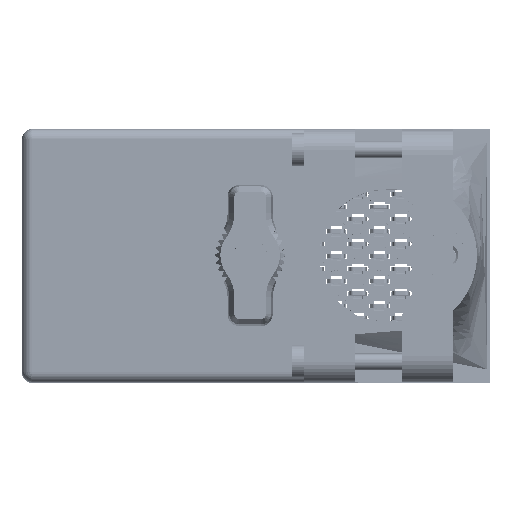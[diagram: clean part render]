
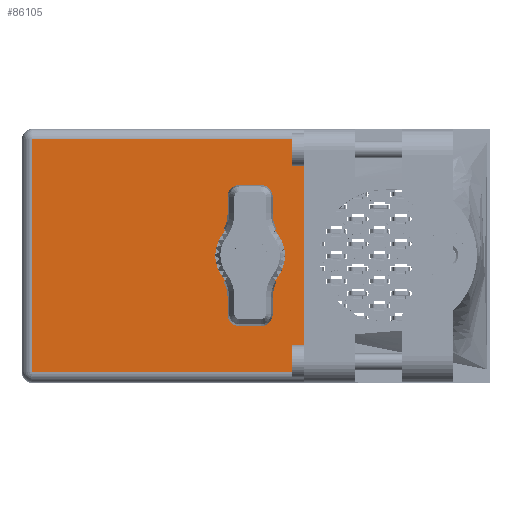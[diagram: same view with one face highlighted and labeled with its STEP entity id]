
A CAD part, top view. The second image highlights one B-rep face of the part: STEP entity #86105.
In plain terms, the highlighted face is planar.
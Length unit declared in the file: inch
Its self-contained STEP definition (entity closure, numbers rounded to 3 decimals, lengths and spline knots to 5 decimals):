
#729 = DIRECTION ( 'NONE',  ( -1., 0., 0. ) ) ;
#3442 = EDGE_CURVE ( 'NONE', #18432, #113699, #70289, .T. ) ;
#4552 = AXIS2_PLACEMENT_3D ( 'NONE', #9886, #89117, #91411 ) ;
#6389 = CIRCLE ( 'NONE', #4552, 0.17 ) ;
#8356 = EDGE_LOOP ( 'NONE', ( #48744, #97580 ) ) ;
#9886 = CARTESIAN_POINT ( 'NONE',  ( 0., 1.93, 0. ) ) ;
#10807 = CARTESIAN_POINT ( 'NONE',  ( 0., 1.93, 0.17 ) ) ;
#12747 = EDGE_CURVE ( 'NONE', #40811, #113699, #49212, .T. ) ;
#14676 = VECTOR ( 'NONE', #64042, 39.37008 ) ;
#18432 = VERTEX_POINT ( 'NONE', #103805 ) ;
#19051 = EDGE_CURVE ( 'NONE', #43180, #21117, #98199, .T. ) ;
#19442 = AXIS2_PLACEMENT_3D ( 'NONE', #82333, #20128, #91129 ) ;
#19872 = EDGE_CURVE ( 'NONE', #21117, #43180, #6389, .T. ) ;
#20128 = DIRECTION ( 'NONE',  ( 0., 1., 0. ) ) ;
#21117 = VERTEX_POINT ( 'NONE', #101809 ) ;
#23657 = FACE_OUTER_BOUND ( 'NONE', #41809, .T. ) ;
#24811 = DIRECTION ( 'NONE',  ( 0., 1., 0. ) ) ;
#25799 = VERTEX_POINT ( 'NONE', #62080 ) ;
#28300 = CARTESIAN_POINT ( 'NONE',  ( -1.3775, 1.93, -0.703 ) ) ;
#29776 = CARTESIAN_POINT ( 'NONE',  ( -1.3155, 1.93, -0.765 ) ) ;
#29930 = CARTESIAN_POINT ( 'NONE',  ( 0.3275, 1.93, 0.703 ) ) ;
#33848 = EDGE_CURVE ( 'NONE', #25799, #40811, #108418, .T. ) ;
#34422 = ORIENTED_EDGE ( 'NONE', *, *, #3442, .F. ) ;
#36672 = CARTESIAN_POINT ( 'NONE',  ( 0.3275, 1.93, 0.703 ) ) ;
#38729 = ORIENTED_EDGE ( 'NONE', *, *, #33848, .T. ) ;
#40124 = VECTOR ( 'NONE', #73173, 39.37008 ) ;
#40266 = EDGE_CURVE ( 'NONE', #18432, #25799, #108667, .T. ) ;
#40811 = VERTEX_POINT ( 'NONE', #93237 ) ;
#41809 = EDGE_LOOP ( 'NONE', ( #38729, #67598, #34422, #82132 ) ) ;
#43180 = VERTEX_POINT ( 'NONE', #10807 ) ;
#43541 = PLANE ( 'NONE',  #76354 ) ;
#45281 = CARTESIAN_POINT ( 'NONE',  ( -1.3775, 1.93, -0.765 ) ) ;
#48744 = ORIENTED_EDGE ( 'NONE', *, *, #19051, .F. ) ;
#49212 = LINE ( 'NONE', #29930, #73661 ) ;
#50764 = VECTOR ( 'NONE', #60319, 39.37008 ) ;
#60319 = DIRECTION ( 'NONE',  ( 0., 0., 1. ) ) ;
#62080 = CARTESIAN_POINT ( 'NONE',  ( -1.3155, 1.93, -0.703 ) ) ;
#62308 = FACE_BOUND ( 'NONE', #8356, .T. ) ;
#64042 = DIRECTION ( 'NONE',  ( -1., 0., 0. ) ) ;
#67598 = ORIENTED_EDGE ( 'NONE', *, *, #12747, .T. ) ;
#70289 = LINE ( 'NONE', #106095, #50764 ) ;
#73173 = DIRECTION ( 'NONE',  ( 0., 0., 1. ) ) ;
#73661 = VECTOR ( 'NONE', #76211, 39.37008 ) ;
#76211 = DIRECTION ( 'NONE',  ( 1., 0., 0. ) ) ;
#76354 = AXIS2_PLACEMENT_3D ( 'NONE', #45281, #24811, #729 ) ;
#82132 = ORIENTED_EDGE ( 'NONE', *, *, #40266, .T. ) ;
#82333 = CARTESIAN_POINT ( 'NONE',  ( 0., 1.93, 0. ) ) ;
#86105 = ADVANCED_FACE ( 'NONE', ( #23657, #62308 ), #43541, .T. ) ;
#89117 = DIRECTION ( 'NONE',  ( 0., 1., 0. ) ) ;
#91129 = DIRECTION ( 'NONE',  ( 0., 0., 1. ) ) ;
#91411 = DIRECTION ( 'NONE',  ( 0., 0., 1. ) ) ;
#93237 = CARTESIAN_POINT ( 'NONE',  ( -1.3155, 1.93, 0.703 ) ) ;
#97580 = ORIENTED_EDGE ( 'NONE', *, *, #19872, .F. ) ;
#98199 = CIRCLE ( 'NONE', #19442, 0.17 ) ;
#101809 = CARTESIAN_POINT ( 'NONE',  ( 0., 1.93, -0.17 ) ) ;
#103805 = CARTESIAN_POINT ( 'NONE',  ( 0.3275, 1.93, -0.703 ) ) ;
#106095 = CARTESIAN_POINT ( 'NONE',  ( 0.3275, 1.93, -0.765 ) ) ;
#108418 = LINE ( 'NONE', #29776, #40124 ) ;
#108667 = LINE ( 'NONE', #28300, #14676 ) ;
#113699 = VERTEX_POINT ( 'NONE', #36672 ) ;
